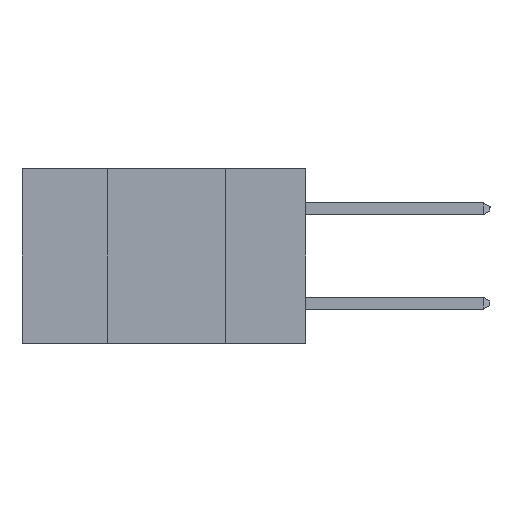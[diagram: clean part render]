
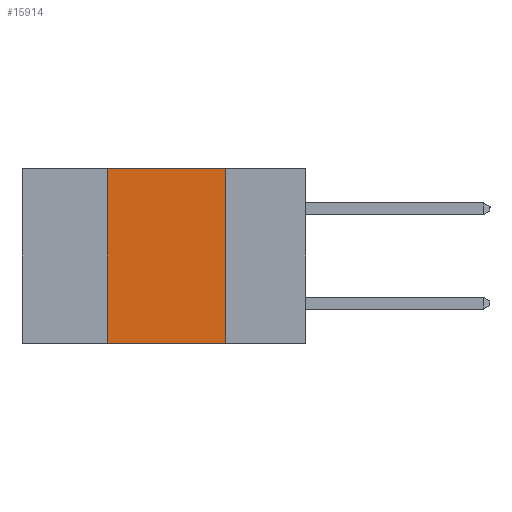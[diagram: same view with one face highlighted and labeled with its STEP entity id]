
A CAD part, left-side view. The second image highlights one B-rep face of the part: STEP entity #15914.
In plain terms, the highlighted planar face has unit normal (-1, 0, 0).
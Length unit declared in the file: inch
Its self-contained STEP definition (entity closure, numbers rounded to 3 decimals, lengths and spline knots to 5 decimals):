
#126 = ORIENTED_EDGE ( 'NONE', *, *, #7960, .F. ) ;
#1005 = ORIENTED_EDGE ( 'NONE', *, *, #9967, .F. ) ;
#1163 = PLANE ( 'NONE',  #8892 ) ;
#1194 = DIRECTION ( 'NONE',  ( 0., -1., 0. ) ) ;
#2577 = VECTOR ( 'NONE', #1194, 39.37008 ) ;
#3303 = VECTOR ( 'NONE', #12260, 39.37008 ) ;
#3505 = LINE ( 'NONE', #8685, #3303 ) ;
#4422 = CARTESIAN_POINT ( 'NONE',  ( 0., 0.42, -0.37 ) ) ;
#4948 = CARTESIAN_POINT ( 'NONE',  ( 0., 0.17, -0.37 ) ) ;
#6694 = DIRECTION ( 'NONE',  ( 0., 0., 1. ) ) ;
#7092 = ORIENTED_EDGE ( 'NONE', *, *, #12091, .T. ) ;
#7738 = VECTOR ( 'NONE', #15261, 39.37008 ) ;
#7960 = EDGE_CURVE ( 'NONE', #9322, #10726, #7982, .T. ) ;
#7982 = LINE ( 'NONE', #11722, #9521 ) ;
#8520 = DIRECTION ( 'NONE',  ( 0., 0., -1. ) ) ;
#8685 = CARTESIAN_POINT ( 'NONE',  ( 0., 0.17, -0.37 ) ) ;
#8842 = VERTEX_POINT ( 'NONE', #9176 ) ;
#8892 = AXIS2_PLACEMENT_3D ( 'NONE', #13585, #12598, #8520 ) ;
#9176 = CARTESIAN_POINT ( 'NONE',  ( 0., 0.17, 0. ) ) ;
#9322 = VERTEX_POINT ( 'NONE', #4422 ) ;
#9521 = VECTOR ( 'NONE', #6694, 39.37008 ) ;
#9710 = LINE ( 'NONE', #13704, #2577 ) ;
#9833 = ORIENTED_EDGE ( 'NONE', *, *, #11951, .F. ) ;
#9967 = EDGE_CURVE ( 'NONE', #8842, #11341, #3505, .T. ) ;
#10726 = VERTEX_POINT ( 'NONE', #13223 ) ;
#11341 = VERTEX_POINT ( 'NONE', #4948 ) ;
#11505 = CARTESIAN_POINT ( 'NONE',  ( 0., 0.6, -0.37 ) ) ;
#11722 = CARTESIAN_POINT ( 'NONE',  ( 0., 0.42, -0.37 ) ) ;
#11951 = EDGE_CURVE ( 'NONE', #10726, #8842, #9710, .T. ) ;
#12091 = EDGE_CURVE ( 'NONE', #9322, #11341, #14275, .T. ) ;
#12260 = DIRECTION ( 'NONE',  ( 0., 0., -1. ) ) ;
#12598 = DIRECTION ( 'NONE',  ( 1., 0., 0. ) ) ;
#13223 = CARTESIAN_POINT ( 'NONE',  ( 0., 0.42, 0. ) ) ;
#13585 = CARTESIAN_POINT ( 'NONE',  ( 0., 0.6, 0. ) ) ;
#13704 = CARTESIAN_POINT ( 'NONE',  ( 0., 0.6, 0. ) ) ;
#13877 = EDGE_LOOP ( 'NONE', ( #1005, #9833, #126, #7092 ) ) ;
#14275 = LINE ( 'NONE', #11505, #7738 ) ;
#14721 = FACE_OUTER_BOUND ( 'NONE', #13877, .T. ) ;
#15261 = DIRECTION ( 'NONE',  ( 0., -1., 0. ) ) ;
#15914 = ADVANCED_FACE ( 'NONE', ( #14721 ), #1163, .F. ) ;
